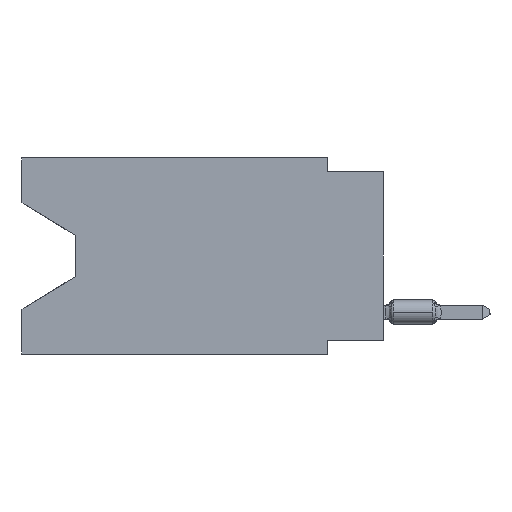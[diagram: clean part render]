
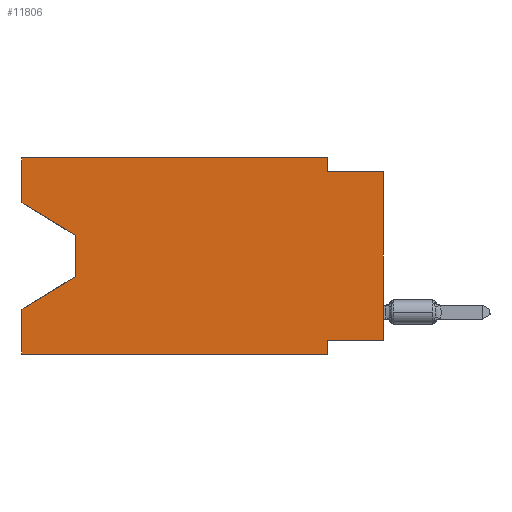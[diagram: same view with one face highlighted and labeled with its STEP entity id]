
A CAD part, left-side view. The second image highlights one B-rep face of the part: STEP entity #11806.
In plain terms, the highlighted planar face has unit normal (-1, 0, 0).
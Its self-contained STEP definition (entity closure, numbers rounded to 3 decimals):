
#1582 = AXIS2_PLACEMENT_3D ( 'NONE', #25163, #24333, #43698 ) ;
#3182 = DIRECTION ( 'NONE',  ( 0., 0., 1. ) ) ;
#4193 = EDGE_CURVE ( 'NONE', #24811, #21976, #34686, .T. ) ;
#5011 = CARTESIAN_POINT ( 'NONE',  ( 0., 16.383, 0. ) ) ;
#6314 = DIRECTION ( 'NONE',  ( 0., 1., 0. ) ) ;
#6616 = VECTOR ( 'NONE', #9808, 1000. ) ;
#7223 = DIRECTION ( 'NONE',  ( 0., -1., 0. ) ) ;
#7415 = CARTESIAN_POINT ( 'NONE',  ( 0., 2.54, -8.89 ) ) ;
#8293 = ORIENTED_EDGE ( 'NONE', *, *, #20026, .T. ) ;
#9298 = EDGE_CURVE ( 'NONE', #43882, #21976, #30389, .T. ) ;
#9764 = VECTOR ( 'NONE', #74851, 1000. ) ;
#9808 = DIRECTION ( 'NONE',  ( 0., 0.855, -0.519 ) ) ;
#10149 = VECTOR ( 'NONE', #47065, 1000. ) ;
#10205 = CARTESIAN_POINT ( 'NONE',  ( 0., 13.97, -5.385 ) ) ;
#10733 = EDGE_LOOP ( 'NONE', ( #46360, #44114, #34494, #17825, #46962, #43987, #54491, #8293, #57976, #41531, #71684, #12754 ) ) ;
#11139 = CARTESIAN_POINT ( 'NONE',  ( 0., 0., -0.635 ) ) ;
#11604 = CARTESIAN_POINT ( 'NONE',  ( 0., 13.97, -3.505 ) ) ;
#11806 = ADVANCED_FACE ( 'NONE', ( #18138 ), #80758, .F. ) ;
#12678 = VERTEX_POINT ( 'NONE', #48505 ) ;
#12719 = VERTEX_POINT ( 'NONE', #31163 ) ;
#12754 = ORIENTED_EDGE ( 'NONE', *, *, #42773, .F. ) ;
#13229 = VECTOR ( 'NONE', #6314, 1000. ) ;
#13853 = VECTOR ( 'NONE', #63874, 1000. ) ;
#14435 = LINE ( 'NONE', #7415, #13853 ) ;
#16990 = DIRECTION ( 'NONE',  ( 0., -1., 0. ) ) ;
#17825 = ORIENTED_EDGE ( 'NONE', *, *, #4193, .F. ) ;
#18138 = FACE_OUTER_BOUND ( 'NONE', #10733, .T. ) ;
#18412 = VERTEX_POINT ( 'NONE', #66578 ) ;
#18715 = LINE ( 'NONE', #55382, #35025 ) ;
#20026 = EDGE_CURVE ( 'NONE', #59318, #26130, #18715, .T. ) ;
#20649 = CARTESIAN_POINT ( 'NONE',  ( 0., 16.383, -6.852 ) ) ;
#21490 = VERTEX_POINT ( 'NONE', #62474 ) ;
#21722 = EDGE_CURVE ( 'NONE', #21996, #18412, #47894, .T. ) ;
#21976 = VERTEX_POINT ( 'NONE', #20649 ) ;
#21996 = VERTEX_POINT ( 'NONE', #72122 ) ;
#22136 = CARTESIAN_POINT ( 'NONE',  ( 0., 0., -8.255 ) ) ;
#24333 = DIRECTION ( 'NONE',  ( 1., 0., 0. ) ) ;
#24811 = VERTEX_POINT ( 'NONE', #30742 ) ;
#25163 = CARTESIAN_POINT ( 'NONE',  ( 0., 16.383, 0. ) ) ;
#26130 = VERTEX_POINT ( 'NONE', #50229 ) ;
#26833 = EDGE_CURVE ( 'NONE', #12678, #43882, #56110, .T. ) ;
#27127 = CARTESIAN_POINT ( 'NONE',  ( 0., 16.383, 0. ) ) ;
#29428 = DIRECTION ( 'NONE',  ( 0., 0., 1. ) ) ;
#30389 = LINE ( 'NONE', #10205, #6616 ) ;
#30742 = CARTESIAN_POINT ( 'NONE',  ( 0., 16.383, -8.89 ) ) ;
#31163 = CARTESIAN_POINT ( 'NONE',  ( 0., 2.54, -8.255 ) ) ;
#33709 = CARTESIAN_POINT ( 'NONE',  ( 0., 16.383, -2.038 ) ) ;
#34494 = ORIENTED_EDGE ( 'NONE', *, *, #9298, .T. ) ;
#34686 = LINE ( 'NONE', #73374, #10149 ) ;
#34913 = DIRECTION ( 'NONE',  ( 0., -0.855, -0.519 ) ) ;
#35025 = VECTOR ( 'NONE', #29428, 1000. ) ;
#36762 = DIRECTION ( 'NONE',  ( 0., 0., -1. ) ) ;
#37645 = LINE ( 'NONE', #62768, #13229 ) ;
#39566 = VECTOR ( 'NONE', #34913, 1000. ) ;
#40298 = LINE ( 'NONE', #33709, #39566 ) ;
#41531 = ORIENTED_EDGE ( 'NONE', *, *, #66697, .F. ) ;
#41875 = CARTESIAN_POINT ( 'NONE',  ( 0., 13.97, -5.385 ) ) ;
#42320 = CARTESIAN_POINT ( 'NONE',  ( 0., 2.54, -0.635 ) ) ;
#42773 = EDGE_CURVE ( 'NONE', #70624, #21996, #72003, .T. ) ;
#42811 = EDGE_CURVE ( 'NONE', #70624, #12678, #40298, .T. ) ;
#43698 = DIRECTION ( 'NONE',  ( 0., 0., -1. ) ) ;
#43882 = VERTEX_POINT ( 'NONE', #41875 ) ;
#43987 = ORIENTED_EDGE ( 'NONE', *, *, #55333, .F. ) ;
#44114 = ORIENTED_EDGE ( 'NONE', *, *, #26833, .T. ) ;
#46360 = ORIENTED_EDGE ( 'NONE', *, *, #42811, .T. ) ;
#46962 = ORIENTED_EDGE ( 'NONE', *, *, #57307, .T. ) ;
#47065 = DIRECTION ( 'NONE',  ( 0., 0., 1. ) ) ;
#47894 = LINE ( 'NONE', #5011, #70768 ) ;
#47956 = EDGE_CURVE ( 'NONE', #81044, #26130, #62237, .T. ) ;
#48505 = CARTESIAN_POINT ( 'NONE',  ( 0., 13.97, -3.505 ) ) ;
#50129 = EDGE_CURVE ( 'NONE', #59318, #12719, #37645, .T. ) ;
#50229 = CARTESIAN_POINT ( 'NONE',  ( 0., 0., -0.635 ) ) ;
#54491 = ORIENTED_EDGE ( 'NONE', *, *, #50129, .F. ) ;
#54900 = VECTOR ( 'NONE', #7223, 1000. ) ;
#55333 = EDGE_CURVE ( 'NONE', #12719, #21490, #14435, .T. ) ;
#55382 = CARTESIAN_POINT ( 'NONE',  ( 0., 0., 0. ) ) ;
#56110 = LINE ( 'NONE', #11604, #59323 ) ;
#56743 = LINE ( 'NONE', #81039, #9764 ) ;
#57307 = EDGE_CURVE ( 'NONE', #24811, #21490, #63681, .T. ) ;
#57976 = ORIENTED_EDGE ( 'NONE', *, *, #47956, .F. ) ;
#59318 = VERTEX_POINT ( 'NONE', #22136 ) ;
#59323 = VECTOR ( 'NONE', #36762, 1000. ) ;
#62237 = LINE ( 'NONE', #11139, #73508 ) ;
#62474 = CARTESIAN_POINT ( 'NONE',  ( 0., 2.54, -8.89 ) ) ;
#62768 = CARTESIAN_POINT ( 'NONE',  ( 0., 0., -8.255 ) ) ;
#63681 = LINE ( 'NONE', #70258, #54900 ) ;
#63874 = DIRECTION ( 'NONE',  ( 0., 0., -1. ) ) ;
#64556 = VECTOR ( 'NONE', #3182, 1000. ) ;
#66578 = CARTESIAN_POINT ( 'NONE',  ( 0., 2.54, 0. ) ) ;
#66697 = EDGE_CURVE ( 'NONE', #18412, #81044, #56743, .T. ) ;
#66795 = DIRECTION ( 'NONE',  ( 0., -1., 0. ) ) ;
#70126 = CARTESIAN_POINT ( 'NONE',  ( 0., 16.383, -2.038 ) ) ;
#70258 = CARTESIAN_POINT ( 'NONE',  ( 0., 16.383, -8.89 ) ) ;
#70624 = VERTEX_POINT ( 'NONE', #70126 ) ;
#70768 = VECTOR ( 'NONE', #16990, 1000. ) ;
#71684 = ORIENTED_EDGE ( 'NONE', *, *, #21722, .F. ) ;
#72003 = LINE ( 'NONE', #27127, #64556 ) ;
#72122 = CARTESIAN_POINT ( 'NONE',  ( 0., 16.383, 0. ) ) ;
#73374 = CARTESIAN_POINT ( 'NONE',  ( 0., 16.383, 0. ) ) ;
#73508 = VECTOR ( 'NONE', #66795, 1000. ) ;
#74851 = DIRECTION ( 'NONE',  ( 0., 0., -1. ) ) ;
#80758 = PLANE ( 'NONE',  #1582 ) ;
#81039 = CARTESIAN_POINT ( 'NONE',  ( 0., 2.54, 0. ) ) ;
#81044 = VERTEX_POINT ( 'NONE', #42320 ) ;
